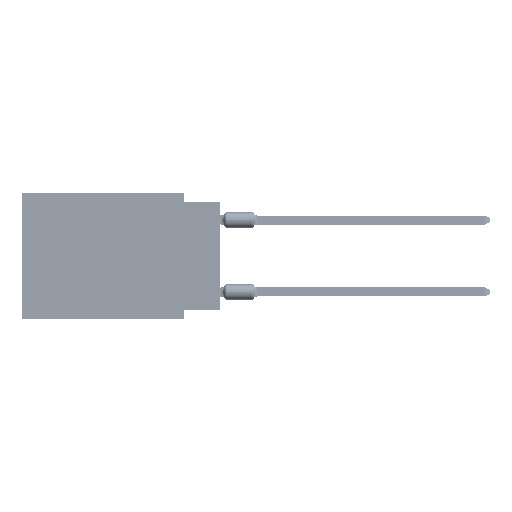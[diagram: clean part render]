
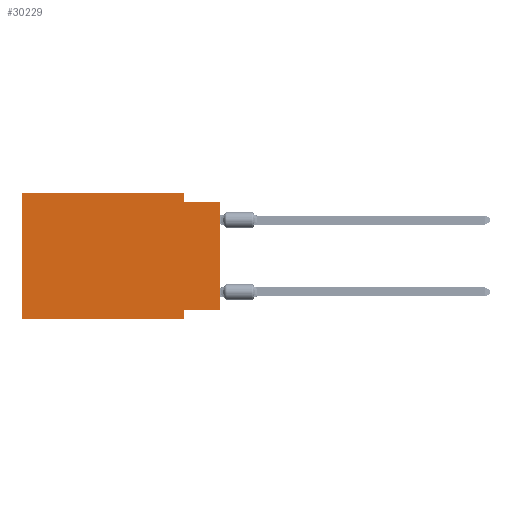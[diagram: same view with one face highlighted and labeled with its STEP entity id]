
A CAD part, left-side view. The second image highlights one B-rep face of the part: STEP entity #30229.
In plain terms, the highlighted planar face has unit normal (-1, 0, 0).
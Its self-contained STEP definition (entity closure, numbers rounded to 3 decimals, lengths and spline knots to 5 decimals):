
#541 = EDGE_CURVE ( 'NONE', #31381, #11108, #68107, .T. ) ;
#721 = VECTOR ( 'NONE', #62522, 39.37008 ) ;
#1696 = CARTESIAN_POINT ( 'NONE',  ( 0., 0.1, -0.025 ) ) ;
#4991 = EDGE_CURVE ( 'NONE', #18698, #59319, #73587, .T. ) ;
#5049 = DIRECTION ( 'NONE',  ( 0., 1., 0. ) ) ;
#7551 = CARTESIAN_POINT ( 'NONE',  ( 0., 0.55, 0. ) ) ;
#8875 = VERTEX_POINT ( 'NONE', #1696 ) ;
#11108 = VERTEX_POINT ( 'NONE', #38101 ) ;
#11276 = CARTESIAN_POINT ( 'NONE',  ( 0., 0.1, 0. ) ) ;
#13620 = DIRECTION ( 'NONE',  ( 0., 0., -1. ) ) ;
#16050 = CARTESIAN_POINT ( 'NONE',  ( 0., 0., -0.025 ) ) ;
#16356 = VERTEX_POINT ( 'NONE', #46614 ) ;
#16410 = LINE ( 'NONE', #38334, #84948 ) ;
#18698 = VERTEX_POINT ( 'NONE', #83480 ) ;
#19212 = EDGE_CURVE ( 'NONE', #8875, #16356, #53834, .T. ) ;
#19409 = VECTOR ( 'NONE', #37235, 39.37008 ) ;
#22734 = CARTESIAN_POINT ( 'NONE',  ( 0., 0., -0.325 ) ) ;
#24979 = LINE ( 'NONE', #7551, #60299 ) ;
#25838 = EDGE_CURVE ( 'NONE', #35663, #16356, #58971, .T. ) ;
#25959 = ORIENTED_EDGE ( 'NONE', *, *, #4991, .F. ) ;
#26500 = CARTESIAN_POINT ( 'NONE',  ( 0., 0., 0. ) ) ;
#29882 = ORIENTED_EDGE ( 'NONE', *, *, #19212, .F. ) ;
#30229 = ADVANCED_FACE ( 'NONE', ( #58009 ), #73665, .F. ) ;
#30411 = CARTESIAN_POINT ( 'NONE',  ( 0., 0.1, -0.325 ) ) ;
#31381 = VERTEX_POINT ( 'NONE', #79960 ) ;
#32342 = ORIENTED_EDGE ( 'NONE', *, *, #25838, .T. ) ;
#33932 = DIRECTION ( 'NONE',  ( 1., 0., 0. ) ) ;
#35663 = VERTEX_POINT ( 'NONE', #22734 ) ;
#36227 = VECTOR ( 'NONE', #78076, 39.37008 ) ;
#37235 = DIRECTION ( 'NONE',  ( 0., 0., -1. ) ) ;
#38101 = CARTESIAN_POINT ( 'NONE',  ( 0., 0.1, -0.35 ) ) ;
#38334 = CARTESIAN_POINT ( 'NONE',  ( 0., 0., -0.325 ) ) ;
#40885 = CARTESIAN_POINT ( 'NONE',  ( 0., 0.55, -0.35 ) ) ;
#41336 = VECTOR ( 'NONE', #53199, 39.37008 ) ;
#44151 = ORIENTED_EDGE ( 'NONE', *, *, #541, .T. ) ;
#44643 = LINE ( 'NONE', #66800, #77819 ) ;
#46614 = CARTESIAN_POINT ( 'NONE',  ( 0., 0., -0.025 ) ) ;
#47468 = DIRECTION ( 'NONE',  ( 0., 0., 1. ) ) ;
#50425 = EDGE_CURVE ( 'NONE', #59319, #8875, #85852, .T. ) ;
#50459 = VECTOR ( 'NONE', #53884, 39.37008 ) ;
#51425 = ORIENTED_EDGE ( 'NONE', *, *, #68803, .F. ) ;
#53199 = DIRECTION ( 'NONE',  ( 0., 0., 1. ) ) ;
#53637 = CARTESIAN_POINT ( 'NONE',  ( 0., 0.55, 0. ) ) ;
#53834 = LINE ( 'NONE', #16050, #721 ) ;
#53884 = DIRECTION ( 'NONE',  ( 0., -1., 0. ) ) ;
#58009 = FACE_OUTER_BOUND ( 'NONE', #81289, .T. ) ;
#58971 = LINE ( 'NONE', #26500, #41336 ) ;
#59319 = VERTEX_POINT ( 'NONE', #80895 ) ;
#60299 = VECTOR ( 'NONE', #47468, 39.37008 ) ;
#62522 = DIRECTION ( 'NONE',  ( 0., -1., 0. ) ) ;
#63113 = ORIENTED_EDGE ( 'NONE', *, *, #76052, .F. ) ;
#63421 = EDGE_CURVE ( 'NONE', #31381, #18698, #24979, .T. ) ;
#64446 = ORIENTED_EDGE ( 'NONE', *, *, #63421, .F. ) ;
#64831 = VERTEX_POINT ( 'NONE', #30411 ) ;
#66800 = CARTESIAN_POINT ( 'NONE',  ( 0., 0.1, -0.35 ) ) ;
#68107 = LINE ( 'NONE', #40885, #50459 ) ;
#68803 = EDGE_CURVE ( 'NONE', #35663, #64831, #16410, .T. ) ;
#73587 = LINE ( 'NONE', #84422, #36227 ) ;
#73665 = PLANE ( 'NONE',  #80231 ) ;
#76052 = EDGE_CURVE ( 'NONE', #64831, #11108, #44643, .T. ) ;
#77819 = VECTOR ( 'NONE', #13620, 39.37008 ) ;
#78076 = DIRECTION ( 'NONE',  ( 0., -1., 0. ) ) ;
#79960 = CARTESIAN_POINT ( 'NONE',  ( 0., 0.55, -0.35 ) ) ;
#80231 = AXIS2_PLACEMENT_3D ( 'NONE', #53637, #33932, #80325 ) ;
#80325 = DIRECTION ( 'NONE',  ( 0., 0., -1. ) ) ;
#80895 = CARTESIAN_POINT ( 'NONE',  ( 0., 0.1, 0. ) ) ;
#80906 = ORIENTED_EDGE ( 'NONE', *, *, #50425, .F. ) ;
#81289 = EDGE_LOOP ( 'NONE', ( #32342, #29882, #80906, #25959, #64446, #44151, #63113, #51425 ) ) ;
#83480 = CARTESIAN_POINT ( 'NONE',  ( 0., 0.55, 0. ) ) ;
#84422 = CARTESIAN_POINT ( 'NONE',  ( 0., 0.55, 0. ) ) ;
#84948 = VECTOR ( 'NONE', #5049, 39.37008 ) ;
#85852 = LINE ( 'NONE', #11276, #19409 ) ;
